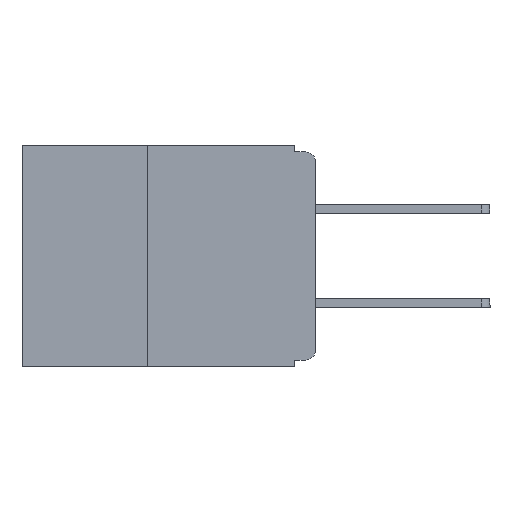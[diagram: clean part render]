
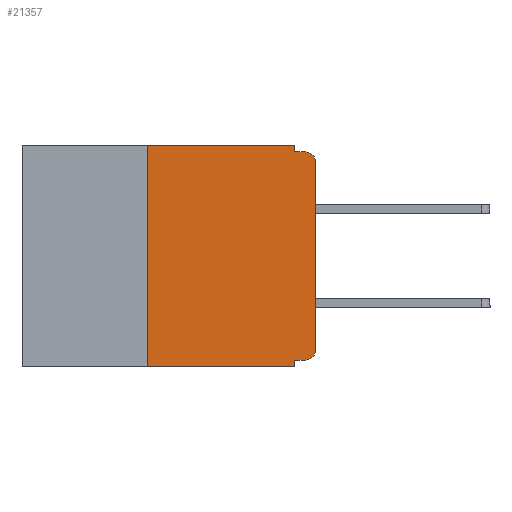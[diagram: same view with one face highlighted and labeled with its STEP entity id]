
A CAD part, left-side view. The second image highlights one B-rep face of the part: STEP entity #21357.
In plain terms, the highlighted planar face has unit normal (-1, 0, 0).
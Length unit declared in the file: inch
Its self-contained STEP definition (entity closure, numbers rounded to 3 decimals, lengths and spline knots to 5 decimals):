
#33 = EDGE_CURVE ( 'NONE', #5330, #8346, #7229, .T. ) ;
#624 = CARTESIAN_POINT ( 'NONE',  ( 0., 0., -0.025 ) ) ;
#686 = DIRECTION ( 'NONE',  ( 0., 0., -1. ) ) ;
#1147 = VECTOR ( 'NONE', #8538, 39.37008 ) ;
#1645 = VERTEX_POINT ( 'NONE', #6776 ) ;
#2915 = VECTOR ( 'NONE', #7975, 39.37008 ) ;
#3240 = EDGE_CURVE ( 'NONE', #24935, #1645, #19668, .T. ) ;
#3303 = DIRECTION ( 'NONE',  ( 0., 0., -1. ) ) ;
#4387 = EDGE_CURVE ( 'NONE', #20863, #5305, #9002, .T. ) ;
#5305 = VERTEX_POINT ( 'NONE', #624 ) ;
#5330 = VERTEX_POINT ( 'NONE', #22893 ) ;
#5797 = CARTESIAN_POINT ( 'NONE',  ( 0., 0., -0.32 ) ) ;
#6487 = ORIENTED_EDGE ( 'NONE', *, *, #33, .F. ) ;
#6744 = ORIENTED_EDGE ( 'NONE', *, *, #10169, .F. ) ;
#6776 = CARTESIAN_POINT ( 'NONE',  ( 0., 0.031, -0.33 ) ) ;
#7229 = LINE ( 'NONE', #15473, #1147 ) ;
#7235 = ORIENTED_EDGE ( 'NONE', *, *, #3240, .T. ) ;
#7412 = EDGE_CURVE ( 'NONE', #5305, #29647, #22299, .T. ) ;
#7975 = DIRECTION ( 'NONE',  ( 0., 0., 1. ) ) ;
#8118 = CARTESIAN_POINT ( 'NONE',  ( 0., 0., 0. ) ) ;
#8304 = ORIENTED_EDGE ( 'NONE', *, *, #30471, .T. ) ;
#8346 = VERTEX_POINT ( 'NONE', #22229 ) ;
#8505 = CARTESIAN_POINT ( 'NONE',  ( 0., 0., -0.01 ) ) ;
#8528 = EDGE_CURVE ( 'NONE', #20420, #29647, #24804, .T. ) ;
#8538 = DIRECTION ( 'NONE',  ( 0., -1., 0. ) ) ;
#9002 = LINE ( 'NONE', #8118, #2915 ) ;
#9064 = CARTESIAN_POINT ( 'NONE',  ( 0., 0.031, -0.32 ) ) ;
#9127 = CARTESIAN_POINT ( 'NONE',  ( 0., 0., -0.305 ) ) ;
#9329 = CARTESIAN_POINT ( 'NONE',  ( 0., 0.031, -0.33 ) ) ;
#10169 = EDGE_CURVE ( 'NONE', #24935, #5330, #29804, .T. ) ;
#10367 = ORIENTED_EDGE ( 'NONE', *, *, #13466, .F. ) ;
#10626 = DIRECTION ( 'NONE',  ( 0., -1., 0. ) ) ;
#10687 = AXIS2_PLACEMENT_3D ( 'NONE', #29915, #15882, #686 ) ;
#10876 = VECTOR ( 'NONE', #24593, 39.37008 ) ;
#11407 = EDGE_LOOP ( 'NONE', ( #25703, #20107, #27603, #10367, #6487, #6744, #7235, #19735, #22496, #8304 ) ) ;
#11415 = DIRECTION ( 'NONE',  ( -1., 0., 0. ) ) ;
#11799 = CARTESIAN_POINT ( 'NONE',  ( 0., 0.437, -0.33 ) ) ;
#12421 = CARTESIAN_POINT ( 'NONE',  ( 0., 0.031, -0.01 ) ) ;
#12834 = DIRECTION ( 'NONE',  ( -1., 0., 0. ) ) ;
#13243 = VERTEX_POINT ( 'NONE', #22060 ) ;
#13279 = VECTOR ( 'NONE', #10626, 39.37008 ) ;
#13466 = EDGE_CURVE ( 'NONE', #8346, #20420, #18091, .T. ) ;
#14615 = VECTOR ( 'NONE', #23660, 39.37008 ) ;
#15473 = CARTESIAN_POINT ( 'NONE',  ( 0., 0.437, 0. ) ) ;
#15758 = EDGE_CURVE ( 'NONE', #13243, #30120, #21271, .T. ) ;
#15878 = CARTESIAN_POINT ( 'NONE',  ( 0., 0.031, 0. ) ) ;
#15882 = DIRECTION ( 'NONE',  ( 1., 0., 0. ) ) ;
#18091 = LINE ( 'NONE', #15878, #29823 ) ;
#18175 = CARTESIAN_POINT ( 'NONE',  ( 0., 0.25, -0.33 ) ) ;
#19668 = LINE ( 'NONE', #11799, #13279 ) ;
#19735 = ORIENTED_EDGE ( 'NONE', *, *, #31400, .F. ) ;
#19874 = AXIS2_PLACEMENT_3D ( 'NONE', #25680, #11415, #28058 ) ;
#20107 = ORIENTED_EDGE ( 'NONE', *, *, #7412, .T. ) ;
#20420 = VERTEX_POINT ( 'NONE', #12421 ) ;
#20863 = VERTEX_POINT ( 'NONE', #9127 ) ;
#21271 = LINE ( 'NONE', #5797, #26795 ) ;
#21357 = ADVANCED_FACE ( 'NONE', ( #26225 ), #25211, .F. ) ;
#21668 = LINE ( 'NONE', #9329, #14615 ) ;
#22060 = CARTESIAN_POINT ( 'NONE',  ( 0., 0.015, -0.32 ) ) ;
#22229 = CARTESIAN_POINT ( 'NONE',  ( 0., 0.031, 0. ) ) ;
#22233 = CARTESIAN_POINT ( 'NONE',  ( 0., 0.25, -0.33 ) ) ;
#22299 = CIRCLE ( 'NONE', #19874, 0.015 ) ;
#22496 = ORIENTED_EDGE ( 'NONE', *, *, #15758, .F. ) ;
#22893 = CARTESIAN_POINT ( 'NONE',  ( 0., 0.25, 0. ) ) ;
#23660 = DIRECTION ( 'NONE',  ( 0., 0., -1. ) ) ;
#23873 = CARTESIAN_POINT ( 'NONE',  ( 0., 0.015, -0.01 ) ) ;
#24593 = DIRECTION ( 'NONE',  ( 0., 0., 1. ) ) ;
#24804 = LINE ( 'NONE', #8505, #25539 ) ;
#24935 = VERTEX_POINT ( 'NONE', #18175 ) ;
#25206 = DIRECTION ( 'NONE',  ( 0., 1., 0. ) ) ;
#25211 = PLANE ( 'NONE',  #10687 ) ;
#25283 = DIRECTION ( 'NONE',  ( 0., -1., 0. ) ) ;
#25539 = VECTOR ( 'NONE', #25283, 39.37008 ) ;
#25680 = CARTESIAN_POINT ( 'NONE',  ( 0., 0.015, -0.025 ) ) ;
#25703 = ORIENTED_EDGE ( 'NONE', *, *, #4387, .T. ) ;
#26153 = AXIS2_PLACEMENT_3D ( 'NONE', #27053, #12834, #29373 ) ;
#26225 = FACE_OUTER_BOUND ( 'NONE', #11407, .T. ) ;
#26795 = VECTOR ( 'NONE', #25206, 39.37008 ) ;
#27053 = CARTESIAN_POINT ( 'NONE',  ( 0., 0.015, -0.305 ) ) ;
#27603 = ORIENTED_EDGE ( 'NONE', *, *, #8528, .F. ) ;
#28058 = DIRECTION ( 'NONE',  ( 0., 0., -1. ) ) ;
#29373 = DIRECTION ( 'NONE',  ( 0., 0., -1. ) ) ;
#29647 = VERTEX_POINT ( 'NONE', #23873 ) ;
#29804 = LINE ( 'NONE', #22233, #10876 ) ;
#29823 = VECTOR ( 'NONE', #3303, 39.37008 ) ;
#29915 = CARTESIAN_POINT ( 'NONE',  ( 0., 0.437, 0. ) ) ;
#30120 = VERTEX_POINT ( 'NONE', #9064 ) ;
#30471 = EDGE_CURVE ( 'NONE', #13243, #20863, #31162, .T. ) ;
#31162 = CIRCLE ( 'NONE', #26153, 0.015 ) ;
#31400 = EDGE_CURVE ( 'NONE', #30120, #1645, #21668, .T. ) ;
